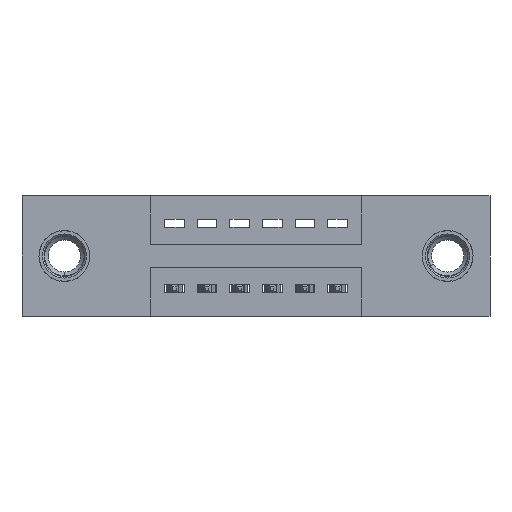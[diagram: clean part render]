
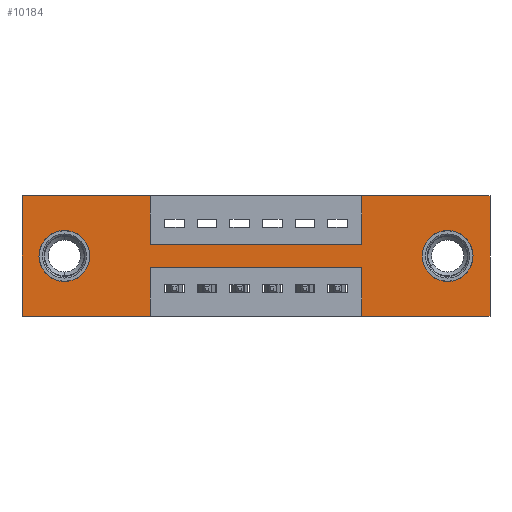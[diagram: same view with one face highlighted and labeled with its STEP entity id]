
A CAD part, front view. The second image highlights one B-rep face of the part: STEP entity #10184.
In plain terms, the highlighted planar face has unit normal (0, -1, 0).
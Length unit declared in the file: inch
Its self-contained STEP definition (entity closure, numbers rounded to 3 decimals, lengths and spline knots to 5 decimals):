
#13 = EDGE_CURVE ( 'NONE', #2290, #809, #6553, .T. ) ;
#52 = CARTESIAN_POINT ( 'NONE',  ( 1.435, 0., 0. ) ) ;
#67 = LINE ( 'NONE', #7182, #7092 ) ;
#89 = DIRECTION ( 'NONE',  ( 0., -1., 0. ) ) ;
#147 = VECTOR ( 'NONE', #6663, 39.37008 ) ;
#204 = ORIENTED_EDGE ( 'NONE', *, *, #7160, .F. ) ;
#380 = EDGE_CURVE ( 'NONE', #2732, #2979, #9548, .T. ) ;
#512 = DIRECTION ( 'NONE',  ( 1., 0., 0. ) ) ;
#601 = EDGE_CURVE ( 'NONE', #4872, #2031, #8115, .T. ) ;
#713 = CARTESIAN_POINT ( 'NONE',  ( 1.305, 0., -0.185 ) ) ;
#777 = ORIENTED_EDGE ( 'NONE', *, *, #9972, .F. ) ;
#809 = VERTEX_POINT ( 'NONE', #52 ) ;
#834 = VECTOR ( 'NONE', #1490, 39.37008 ) ;
#852 = LINE ( 'NONE', #4243, #2951 ) ;
#883 = VERTEX_POINT ( 'NONE', #3140 ) ;
#916 = VERTEX_POINT ( 'NONE', #7127 ) ;
#1054 = ORIENTED_EDGE ( 'NONE', *, *, #7281, .T. ) ;
#1057 = CARTESIAN_POINT ( 'NONE',  ( 0.3925, 0., -0.37 ) ) ;
#1071 = ORIENTED_EDGE ( 'NONE', *, *, #5071, .F. ) ;
#1092 = LINE ( 'NONE', #4090, #7458 ) ;
#1144 = VECTOR ( 'NONE', #8142, 39.37008 ) ;
#1337 = EDGE_CURVE ( 'NONE', #4252, #8000, #4518, .T. ) ;
#1382 = DIRECTION ( 'NONE',  ( 0., 0., -1. ) ) ;
#1443 = LINE ( 'NONE', #10380, #1144 ) ;
#1490 = DIRECTION ( 'NONE',  ( 0., 0., -1. ) ) ;
#1548 = CARTESIAN_POINT ( 'NONE',  ( 0., 0., -0.37 ) ) ;
#1610 = VERTEX_POINT ( 'NONE', #1548 ) ;
#1679 = ORIENTED_EDGE ( 'NONE', *, *, #380, .T. ) ;
#1885 = CARTESIAN_POINT ( 'NONE',  ( 1.305, 0., -0.185 ) ) ;
#1895 = ORIENTED_EDGE ( 'NONE', *, *, #7880, .T. ) ;
#2031 = VERTEX_POINT ( 'NONE', #5376 ) ;
#2066 = LINE ( 'NONE', #5239, #10275 ) ;
#2071 = DIRECTION ( 'NONE',  ( 1., 0., 0. ) ) ;
#2080 = EDGE_CURVE ( 'NONE', #8000, #2290, #2066, .T. ) ;
#2103 = AXIS2_PLACEMENT_3D ( 'NONE', #9905, #89, #6100 ) ;
#2153 = CARTESIAN_POINT ( 'NONE',  ( 1.305, 0., -0.263 ) ) ;
#2225 = LINE ( 'NONE', #2968, #10189 ) ;
#2290 = VERTEX_POINT ( 'NONE', #4141 ) ;
#2559 = LINE ( 'NONE', #5888, #147 ) ;
#2567 = ORIENTED_EDGE ( 'NONE', *, *, #10416, .F. ) ;
#2603 = EDGE_LOOP ( 'NONE', ( #7948, #204, #777, #8885, #8757, #5193, #2839, #4335, #4704, #2567, #4685, #1071 ) ) ;
#2732 = VERTEX_POINT ( 'NONE', #9374 ) ;
#2760 = DIRECTION ( 'NONE',  ( 0., 0., -1. ) ) ;
#2822 = CARTESIAN_POINT ( 'NONE',  ( 0., 0., 0. ) ) ;
#2839 = ORIENTED_EDGE ( 'NONE', *, *, #2080, .F. ) ;
#2879 = VERTEX_POINT ( 'NONE', #7679 ) ;
#2910 = CARTESIAN_POINT ( 'NONE',  ( 1.0425, 0., -0.15 ) ) ;
#2951 = VECTOR ( 'NONE', #7399, 39.37008 ) ;
#2968 = CARTESIAN_POINT ( 'NONE',  ( 0.3925, 0., -0.22 ) ) ;
#2979 = VERTEX_POINT ( 'NONE', #3165 ) ;
#3140 = CARTESIAN_POINT ( 'NONE',  ( 1.435, 0., -0.37 ) ) ;
#3154 = LINE ( 'NONE', #10261, #5117 ) ;
#3160 = CIRCLE ( 'NONE', #4229, 0.078 ) ;
#3165 = CARTESIAN_POINT ( 'NONE',  ( 0.13, 0., -0.263 ) ) ;
#3559 = CIRCLE ( 'NONE', #8068, 0.078 ) ;
#3803 = ORIENTED_EDGE ( 'NONE', *, *, #601, .T. ) ;
#3831 = CARTESIAN_POINT ( 'NONE',  ( 0.3925, 0., 0. ) ) ;
#3841 = DIRECTION ( 'NONE',  ( -1., 0., 0. ) ) ;
#4090 = CARTESIAN_POINT ( 'NONE',  ( 1.0425, 0., -0.37 ) ) ;
#4103 = CARTESIAN_POINT ( 'NONE',  ( 0.3925, 0., -0.37 ) ) ;
#4141 = CARTESIAN_POINT ( 'NONE',  ( 1.0425, 0., 0. ) ) ;
#4229 = AXIS2_PLACEMENT_3D ( 'NONE', #9127, #4426, #9880 ) ;
#4243 = CARTESIAN_POINT ( 'NONE',  ( 0., 0., 0. ) ) ;
#4252 = VERTEX_POINT ( 'NONE', #7585 ) ;
#4261 = VECTOR ( 'NONE', #9324, 39.37008 ) ;
#4335 = ORIENTED_EDGE ( 'NONE', *, *, #1337, .F. ) ;
#4426 = DIRECTION ( 'NONE',  ( 0., 1., 0. ) ) ;
#4484 = EDGE_CURVE ( 'NONE', #883, #8609, #2559, .T. ) ;
#4518 = LINE ( 'NONE', #9060, #6414 ) ;
#4634 = CARTESIAN_POINT ( 'NONE',  ( 0.13, 0., -0.185 ) ) ;
#4685 = ORIENTED_EDGE ( 'NONE', *, *, #5127, .F. ) ;
#4704 = ORIENTED_EDGE ( 'NONE', *, *, #9120, .F. ) ;
#4803 = CARTESIAN_POINT ( 'NONE',  ( 1.0425, 0., -0.37 ) ) ;
#4872 = VERTEX_POINT ( 'NONE', #2153 ) ;
#4974 = EDGE_LOOP ( 'NONE', ( #1895, #3803 ) ) ;
#5071 = EDGE_CURVE ( 'NONE', #7343, #1610, #1443, .T. ) ;
#5117 = VECTOR ( 'NONE', #512, 39.37008 ) ;
#5127 = EDGE_CURVE ( 'NONE', #1610, #9847, #852, .T. ) ;
#5193 = ORIENTED_EDGE ( 'NONE', *, *, #13, .F. ) ;
#5239 = CARTESIAN_POINT ( 'NONE',  ( 1.0425, 0., 0. ) ) ;
#5311 = PLANE ( 'NONE',  #2103 ) ;
#5376 = CARTESIAN_POINT ( 'NONE',  ( 1.305, 0., -0.107 ) ) ;
#5420 = DIRECTION ( 'NONE',  ( 0., 0., 1. ) ) ;
#5432 = AXIS2_PLACEMENT_3D ( 'NONE', #4634, #8229, #8325 ) ;
#5888 = CARTESIAN_POINT ( 'NONE',  ( 0., 0., -0.37 ) ) ;
#6100 = DIRECTION ( 'NONE',  ( 0., 0., -1. ) ) ;
#6414 = VECTOR ( 'NONE', #8575, 39.37008 ) ;
#6553 = LINE ( 'NONE', #2822, #8372 ) ;
#6637 = LINE ( 'NONE', #3831, #4261 ) ;
#6663 = DIRECTION ( 'NONE',  ( -1., 0., 0. ) ) ;
#6936 = CARTESIAN_POINT ( 'NONE',  ( 0.3925, 0., 0. ) ) ;
#7092 = VECTOR ( 'NONE', #1382, 39.37008 ) ;
#7127 = CARTESIAN_POINT ( 'NONE',  ( 0.3925, 0., -0.22 ) ) ;
#7160 = EDGE_CURVE ( 'NONE', #2879, #916, #2225, .T. ) ;
#7182 = CARTESIAN_POINT ( 'NONE',  ( 1.435, 0., 0. ) ) ;
#7281 = EDGE_CURVE ( 'NONE', #2979, #2732, #3160, .T. ) ;
#7343 = VERTEX_POINT ( 'NONE', #1057 ) ;
#7399 = DIRECTION ( 'NONE',  ( 0., 0., 1. ) ) ;
#7458 = VECTOR ( 'NONE', #8027, 39.37008 ) ;
#7542 = EDGE_CURVE ( 'NONE', #809, #883, #67, .T. ) ;
#7580 = FACE_OUTER_BOUND ( 'NONE', #2603, .T. ) ;
#7585 = CARTESIAN_POINT ( 'NONE',  ( 0.3925, 0., -0.15 ) ) ;
#7612 = DIRECTION ( 'NONE',  ( 0., 1., 0. ) ) ;
#7679 = CARTESIAN_POINT ( 'NONE',  ( 1.0425, 0., -0.22 ) ) ;
#7728 = LINE ( 'NONE', #4103, #834 ) ;
#7814 = FACE_BOUND ( 'NONE', #10514, .T. ) ;
#7880 = EDGE_CURVE ( 'NONE', #2031, #4872, #3559, .T. ) ;
#7942 = CARTESIAN_POINT ( 'NONE',  ( 0., 0., 0. ) ) ;
#7948 = ORIENTED_EDGE ( 'NONE', *, *, #8213, .F. ) ;
#7966 = VERTEX_POINT ( 'NONE', #6936 ) ;
#8000 = VERTEX_POINT ( 'NONE', #2910 ) ;
#8027 = DIRECTION ( 'NONE',  ( 0., 0., 1. ) ) ;
#8068 = AXIS2_PLACEMENT_3D ( 'NONE', #1885, #7612, #2760 ) ;
#8115 = CIRCLE ( 'NONE', #10105, 0.078 ) ;
#8142 = DIRECTION ( 'NONE',  ( -1., 0., 0. ) ) ;
#8213 = EDGE_CURVE ( 'NONE', #916, #7343, #7728, .T. ) ;
#8229 = DIRECTION ( 'NONE',  ( 0., 1., 0. ) ) ;
#8325 = DIRECTION ( 'NONE',  ( 0., 0., 1. ) ) ;
#8372 = VECTOR ( 'NONE', #2071, 39.37008 ) ;
#8575 = DIRECTION ( 'NONE',  ( 1., 0., 0. ) ) ;
#8609 = VERTEX_POINT ( 'NONE', #4803 ) ;
#8757 = ORIENTED_EDGE ( 'NONE', *, *, #7542, .F. ) ;
#8885 = ORIENTED_EDGE ( 'NONE', *, *, #4484, .F. ) ;
#9060 = CARTESIAN_POINT ( 'NONE',  ( 0.3925, 0., -0.15 ) ) ;
#9120 = EDGE_CURVE ( 'NONE', #7966, #4252, #6637, .T. ) ;
#9127 = CARTESIAN_POINT ( 'NONE',  ( 0.13, 0., -0.185 ) ) ;
#9324 = DIRECTION ( 'NONE',  ( 0., 0., -1. ) ) ;
#9374 = CARTESIAN_POINT ( 'NONE',  ( 0.13, 0., -0.107 ) ) ;
#9548 = CIRCLE ( 'NONE', #5432, 0.078 ) ;
#9606 = FACE_BOUND ( 'NONE', #4974, .T. ) ;
#9847 = VERTEX_POINT ( 'NONE', #7942 ) ;
#9880 = DIRECTION ( 'NONE',  ( 0., 0., 1. ) ) ;
#9905 = CARTESIAN_POINT ( 'NONE',  ( 0., 0., -0.37 ) ) ;
#9972 = EDGE_CURVE ( 'NONE', #8609, #2879, #1092, .T. ) ;
#10077 = DIRECTION ( 'NONE',  ( 0., 0., -1. ) ) ;
#10105 = AXIS2_PLACEMENT_3D ( 'NONE', #713, #10312, #10077 ) ;
#10184 = ADVANCED_FACE ( 'NONE', ( #9606, #7814, #7580 ), #5311, .T. ) ;
#10189 = VECTOR ( 'NONE', #3841, 39.37008 ) ;
#10261 = CARTESIAN_POINT ( 'NONE',  ( 0., 0., 0. ) ) ;
#10275 = VECTOR ( 'NONE', #5420, 39.37008 ) ;
#10312 = DIRECTION ( 'NONE',  ( 0., 1., 0. ) ) ;
#10380 = CARTESIAN_POINT ( 'NONE',  ( 0., 0., -0.37 ) ) ;
#10416 = EDGE_CURVE ( 'NONE', #9847, #7966, #3154, .T. ) ;
#10514 = EDGE_LOOP ( 'NONE', ( #1679, #1054 ) ) ;
